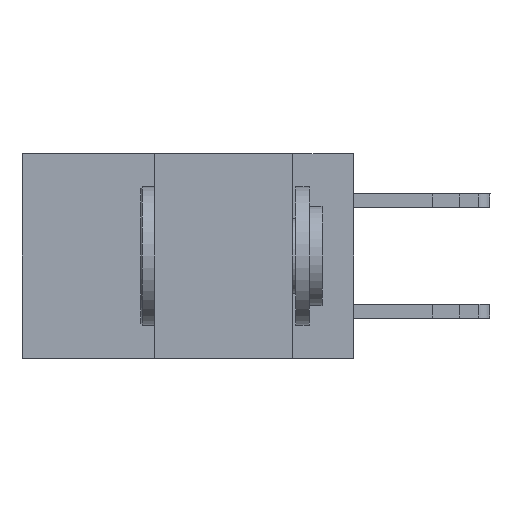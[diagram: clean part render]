
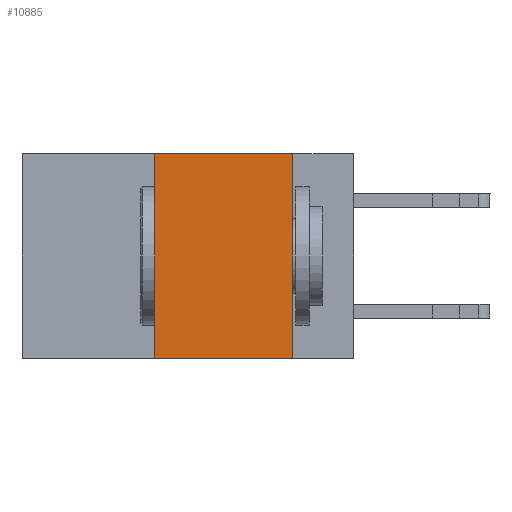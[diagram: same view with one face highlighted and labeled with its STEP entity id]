
A CAD part, left-side view. The second image highlights one B-rep face of the part: STEP entity #10885.
In plain terms, the highlighted planar face has unit normal (-1, 0, 0).
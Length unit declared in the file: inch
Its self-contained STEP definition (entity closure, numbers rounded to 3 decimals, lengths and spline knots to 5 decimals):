
#256 = CARTESIAN_POINT ( 'NONE',  ( 0., 0.36, 0. ) ) ;
#666 = CARTESIAN_POINT ( 'NONE',  ( 0., 0.6, 0. ) ) ;
#1363 = VECTOR ( 'NONE', #4829, 39.37008 ) ;
#1913 = LINE ( 'NONE', #16391, #8424 ) ;
#2443 = CARTESIAN_POINT ( 'NONE',  ( 0., 0.11, 0. ) ) ;
#4158 = ORIENTED_EDGE ( 'NONE', *, *, #8420, .F. ) ;
#4180 = ORIENTED_EDGE ( 'NONE', *, *, #14262, .F. ) ;
#4829 = DIRECTION ( 'NONE',  ( 0., -1., 0. ) ) ;
#5116 = DIRECTION ( 'NONE',  ( 0., 0., 1. ) ) ;
#5519 = LINE ( 'NONE', #20032, #1363 ) ;
#6327 = PLANE ( 'NONE',  #17970 ) ;
#8420 = EDGE_CURVE ( 'NONE', #14615, #10603, #5519, .T. ) ;
#8424 = VECTOR ( 'NONE', #12675, 39.37008 ) ;
#9458 = CARTESIAN_POINT ( 'NONE',  ( 0., 0.6, -0.37 ) ) ;
#9805 = VECTOR ( 'NONE', #5116, 39.37008 ) ;
#9877 = DIRECTION ( 'NONE',  ( 1., 0., 0. ) ) ;
#10453 = VERTEX_POINT ( 'NONE', #19239 ) ;
#10603 = VERTEX_POINT ( 'NONE', #2443 ) ;
#10706 = FACE_OUTER_BOUND ( 'NONE', #19957, .T. ) ;
#10885 = ADVANCED_FACE ( 'NONE', ( #10706 ), #6327, .F. ) ;
#10972 = CARTESIAN_POINT ( 'NONE',  ( 0., 0.11, -0.37 ) ) ;
#11900 = ORIENTED_EDGE ( 'NONE', *, *, #21982, .F. ) ;
#12675 = DIRECTION ( 'NONE',  ( 0., 0., -1. ) ) ;
#13275 = DIRECTION ( 'NONE',  ( 0., -1., 0. ) ) ;
#13566 = LINE ( 'NONE', #9458, #24264 ) ;
#13963 = DIRECTION ( 'NONE',  ( 0., 0., -1. ) ) ;
#14262 = EDGE_CURVE ( 'NONE', #10603, #16878, #1913, .T. ) ;
#14483 = EDGE_CURVE ( 'NONE', #10453, #16878, #13566, .T. ) ;
#14571 = CARTESIAN_POINT ( 'NONE',  ( 0., 0.36, 0. ) ) ;
#14615 = VERTEX_POINT ( 'NONE', #256 ) ;
#16391 = CARTESIAN_POINT ( 'NONE',  ( 0., 0.11, 0. ) ) ;
#16878 = VERTEX_POINT ( 'NONE', #10972 ) ;
#17970 = AXIS2_PLACEMENT_3D ( 'NONE', #666, #9877, #13963 ) ;
#19239 = CARTESIAN_POINT ( 'NONE',  ( 0., 0.36, -0.37 ) ) ;
#19872 = LINE ( 'NONE', #14571, #9805 ) ;
#19957 = EDGE_LOOP ( 'NONE', ( #4180, #4158, #11900, #20426 ) ) ;
#20032 = CARTESIAN_POINT ( 'NONE',  ( 0., 0.6, 0. ) ) ;
#20426 = ORIENTED_EDGE ( 'NONE', *, *, #14483, .T. ) ;
#21982 = EDGE_CURVE ( 'NONE', #10453, #14615, #19872, .T. ) ;
#24264 = VECTOR ( 'NONE', #13275, 39.37008 ) ;
